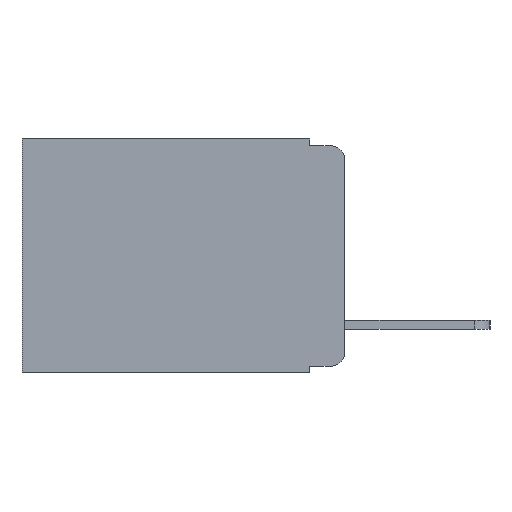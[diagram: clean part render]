
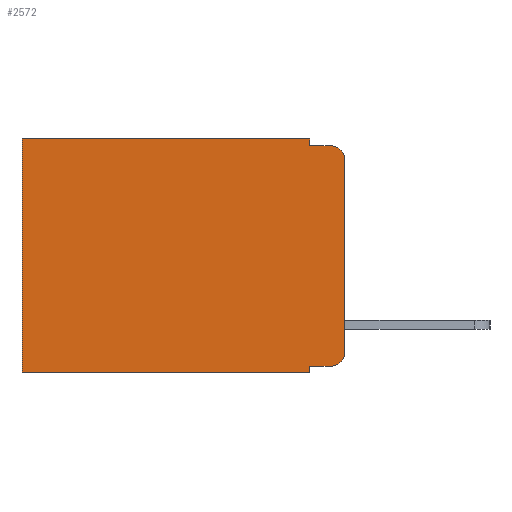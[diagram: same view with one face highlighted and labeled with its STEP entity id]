
A CAD part, left-side view. The second image highlights one B-rep face of the part: STEP entity #2572.
In plain terms, the highlighted planar face has unit normal (-1, 0, 0).
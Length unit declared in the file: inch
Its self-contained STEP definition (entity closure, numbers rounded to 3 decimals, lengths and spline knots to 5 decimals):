
#73 = CIRCLE ( 'NONE', #3098, 0.02 ) ;
#233 = CARTESIAN_POINT ( 'NONE',  ( 0.298, 0., 0. ) ) ;
#481 = VERTEX_POINT ( 'NONE', #9599 ) ;
#618 = ORIENTED_EDGE ( 'NONE', *, *, #2915, .F. ) ;
#715 = CARTESIAN_POINT ( 'NONE',  ( 0.298, 0.473, 0. ) ) ;
#761 = ORIENTED_EDGE ( 'NONE', *, *, #3392, .F. ) ;
#829 = CARTESIAN_POINT ( 'NONE',  ( 0.298, 0.02, -0.313 ) ) ;
#858 = VECTOR ( 'NONE', #1693, 39.37008 ) ;
#949 = DIRECTION ( 'NONE',  ( -1., 0., 0. ) ) ;
#1215 = LINE ( 'NONE', #9593, #858 ) ;
#1289 = ORIENTED_EDGE ( 'NONE', *, *, #3358, .F. ) ;
#1344 = DIRECTION ( 'NONE',  ( 0., -1., 0. ) ) ;
#1418 = VERTEX_POINT ( 'NONE', #10852 ) ;
#1468 = DIRECTION ( 'NONE',  ( 0., 0., -1. ) ) ;
#1541 = AXIS2_PLACEMENT_3D ( 'NONE', #7298, #11028, #5686 ) ;
#1693 = DIRECTION ( 'NONE',  ( 0., 1., 0. ) ) ;
#1695 = VERTEX_POINT ( 'NONE', #6988 ) ;
#1827 = EDGE_CURVE ( 'NONE', #1418, #7137, #4956, .T. ) ;
#2158 = ORIENTED_EDGE ( 'NONE', *, *, #3458, .T. ) ;
#2284 = CARTESIAN_POINT ( 'NONE',  ( 0.298, 0.02, -0.333 ) ) ;
#2404 = CARTESIAN_POINT ( 'NONE',  ( 0.298, 0.051, 0. ) ) ;
#2572 = ADVANCED_FACE ( 'NONE', ( #8375 ), #8252, .F. ) ;
#2706 = CARTESIAN_POINT ( 'NONE',  ( 0.298, 0., 0. ) ) ;
#2915 = EDGE_CURVE ( 'NONE', #6710, #3656, #1215, .T. ) ;
#3020 = ORIENTED_EDGE ( 'NONE', *, *, #3389, .T. ) ;
#3098 = AXIS2_PLACEMENT_3D ( 'NONE', #829, #949, #1468 ) ;
#3358 = EDGE_CURVE ( 'NONE', #9678, #1695, #9598, .T. ) ;
#3389 = EDGE_CURVE ( 'NONE', #9678, #481, #6800, .T. ) ;
#3392 = EDGE_CURVE ( 'NONE', #11751, #481, #8857, .T. ) ;
#3395 = LINE ( 'NONE', #7316, #10214 ) ;
#3407 = EDGE_CURVE ( 'NONE', #1418, #11751, #8602, .T. ) ;
#3458 = EDGE_CURVE ( 'NONE', #7137, #3656, #10465, .T. ) ;
#3463 = EDGE_CURVE ( 'NONE', #6396, #6710, #3395, .T. ) ;
#3481 = EDGE_CURVE ( 'NONE', #6396, #7293, #8046, .T. ) ;
#3483 = EDGE_CURVE ( 'NONE', #7293, #1695, #73, .T. ) ;
#3519 = ORIENTED_EDGE ( 'NONE', *, *, #1827, .T. ) ;
#3656 = VERTEX_POINT ( 'NONE', #11136 ) ;
#3670 = DIRECTION ( 'NONE',  ( 0., 1., 0. ) ) ;
#3715 = VECTOR ( 'NONE', #11546, 39.37008 ) ;
#3966 = DIRECTION ( 'NONE',  ( 0., 0., -1. ) ) ;
#4577 = VECTOR ( 'NONE', #6421, 39.37008 ) ;
#4956 = LINE ( 'NONE', #233, #11780 ) ;
#5112 = CARTESIAN_POINT ( 'NONE',  ( 0.298, 0.051, -0.343 ) ) ;
#5334 = VECTOR ( 'NONE', #1344, 39.37008 ) ;
#5646 = CARTESIAN_POINT ( 'NONE',  ( 0.298, 0.051, -0.01 ) ) ;
#5686 = DIRECTION ( 'NONE',  ( 0., 0., -1. ) ) ;
#5797 = CARTESIAN_POINT ( 'NONE',  ( 0.298, 0.473, 0. ) ) ;
#5855 = AXIS2_PLACEMENT_3D ( 'NONE', #2706, #5918, #6226 ) ;
#5887 = DIRECTION ( 'NONE',  ( 0., 0., -1. ) ) ;
#5918 = DIRECTION ( 'NONE',  ( 1., 0., 0. ) ) ;
#6226 = DIRECTION ( 'NONE',  ( 0., 0., -1. ) ) ;
#6237 = VECTOR ( 'NONE', #3966, 39.37008 ) ;
#6396 = VERTEX_POINT ( 'NONE', #10568 ) ;
#6421 = DIRECTION ( 'NONE',  ( 0., 0., -1. ) ) ;
#6514 = VECTOR ( 'NONE', #6604, 39.37008 ) ;
#6555 = ORIENTED_EDGE ( 'NONE', *, *, #3483, .T. ) ;
#6604 = DIRECTION ( 'NONE',  ( 0., -1., 0. ) ) ;
#6625 = ORIENTED_EDGE ( 'NONE', *, *, #3481, .T. ) ;
#6710 = VERTEX_POINT ( 'NONE', #5112 ) ;
#6800 = CIRCLE ( 'NONE', #1541, 0.02 ) ;
#6988 = CARTESIAN_POINT ( 'NONE',  ( 0.298, 0., -0.313 ) ) ;
#7137 = VERTEX_POINT ( 'NONE', #715 ) ;
#7204 = ORIENTED_EDGE ( 'NONE', *, *, #3463, .F. ) ;
#7293 = VERTEX_POINT ( 'NONE', #2284 ) ;
#7298 = CARTESIAN_POINT ( 'NONE',  ( 0.298, 0.02, -0.03 ) ) ;
#7316 = CARTESIAN_POINT ( 'NONE',  ( 0.298, 0.051, 0. ) ) ;
#7816 = EDGE_LOOP ( 'NONE', ( #1289, #3020, #761, #11571, #3519, #2158, #618, #7204, #6625, #6555 ) ) ;
#8046 = LINE ( 'NONE', #11292, #5334 ) ;
#8252 = PLANE ( 'NONE',  #5855 ) ;
#8375 = FACE_OUTER_BOUND ( 'NONE', #7816, .T. ) ;
#8602 = LINE ( 'NONE', #2404, #6237 ) ;
#8857 = LINE ( 'NONE', #9564, #6514 ) ;
#9564 = CARTESIAN_POINT ( 'NONE',  ( 0.298, 0.051, -0.01 ) ) ;
#9593 = CARTESIAN_POINT ( 'NONE',  ( 0.298, 0., -0.343 ) ) ;
#9598 = LINE ( 'NONE', #10358, #4577 ) ;
#9599 = CARTESIAN_POINT ( 'NONE',  ( 0.298, 0.02, -0.01 ) ) ;
#9678 = VERTEX_POINT ( 'NONE', #9862 ) ;
#9862 = CARTESIAN_POINT ( 'NONE',  ( 0.298, 0., -0.03 ) ) ;
#10214 = VECTOR ( 'NONE', #5887, 39.37008 ) ;
#10358 = CARTESIAN_POINT ( 'NONE',  ( 0.298, 0., 0. ) ) ;
#10465 = LINE ( 'NONE', #5797, #3715 ) ;
#10568 = CARTESIAN_POINT ( 'NONE',  ( 0.298, 0.051, -0.333 ) ) ;
#10852 = CARTESIAN_POINT ( 'NONE',  ( 0.298, 0.051, 0. ) ) ;
#11028 = DIRECTION ( 'NONE',  ( -1., 0., 0. ) ) ;
#11136 = CARTESIAN_POINT ( 'NONE',  ( 0.298, 0.473, -0.343 ) ) ;
#11292 = CARTESIAN_POINT ( 'NONE',  ( 0.298, 0.051, -0.333 ) ) ;
#11546 = DIRECTION ( 'NONE',  ( 0., 0., -1. ) ) ;
#11571 = ORIENTED_EDGE ( 'NONE', *, *, #3407, .F. ) ;
#11751 = VERTEX_POINT ( 'NONE', #5646 ) ;
#11780 = VECTOR ( 'NONE', #3670, 39.37008 ) ;
